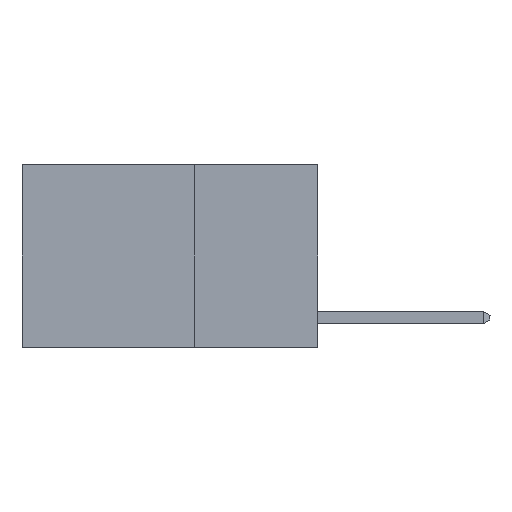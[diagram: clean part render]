
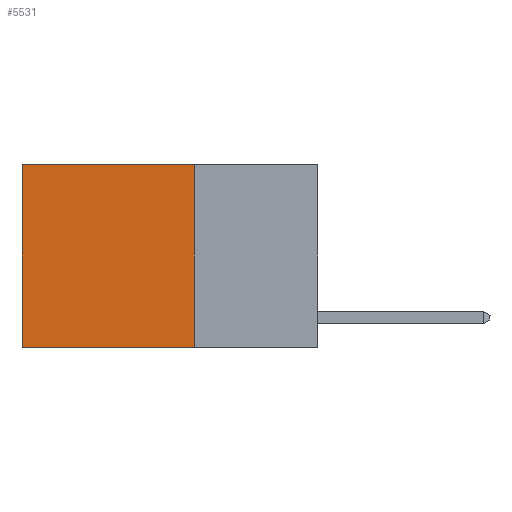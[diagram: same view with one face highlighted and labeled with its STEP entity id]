
A CAD part, left-side view. The second image highlights one B-rep face of the part: STEP entity #5531.
In plain terms, the highlighted planar face has unit normal (-1, 0, 0).
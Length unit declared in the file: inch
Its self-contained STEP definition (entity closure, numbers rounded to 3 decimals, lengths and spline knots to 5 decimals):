
#133 = LINE ( 'NONE', #4720, #2560 ) ;
#570 = EDGE_CURVE ( 'NONE', #7562, #9712, #12579, .T. ) ;
#711 = CARTESIAN_POINT ( 'NONE',  ( 0.2625, 0.6, 0. ) ) ;
#1269 = CARTESIAN_POINT ( 'NONE',  ( 0.2625, 0.6, -0.37 ) ) ;
#2114 = EDGE_CURVE ( 'NONE', #3166, #11554, #12125, .T. ) ;
#2398 = DIRECTION ( 'NONE',  ( 0., 0., -1. ) ) ;
#2560 = VECTOR ( 'NONE', #13889, 39.37008 ) ;
#3121 = DIRECTION ( 'NONE',  ( 0., 0., -1. ) ) ;
#3166 = VERTEX_POINT ( 'NONE', #5703 ) ;
#3882 = DIRECTION ( 'NONE',  ( 0., 1., 0. ) ) ;
#3989 = VECTOR ( 'NONE', #3121, 39.37008 ) ;
#4628 = PLANE ( 'NONE',  #12241 ) ;
#4720 = CARTESIAN_POINT ( 'NONE',  ( 0.2625, 0.25, -0.37 ) ) ;
#5531 = ADVANCED_FACE ( 'NONE', ( #12671 ), #4628, .F. ) ;
#5702 = EDGE_CURVE ( 'NONE', #7562, #3166, #8377, .T. ) ;
#5703 = CARTESIAN_POINT ( 'NONE',  ( 0.2625, 0.6, 0. ) ) ;
#5967 = CARTESIAN_POINT ( 'NONE',  ( 0.2625, 0.25, 0. ) ) ;
#6939 = CARTESIAN_POINT ( 'NONE',  ( 0.2625, 0.25, 0. ) ) ;
#7374 = EDGE_LOOP ( 'NONE', ( #14693, #11325, #11069, #13743 ) ) ;
#7562 = VERTEX_POINT ( 'NONE', #9446 ) ;
#7916 = DIRECTION ( 'NONE',  ( 0., 0., -1. ) ) ;
#8128 = VECTOR ( 'NONE', #3882, 39.37008 ) ;
#8377 = LINE ( 'NONE', #9724, #8128 ) ;
#8562 = VECTOR ( 'NONE', #7916, 39.37008 ) ;
#9446 = CARTESIAN_POINT ( 'NONE',  ( 0.2625, 0.25, 0. ) ) ;
#9712 = VERTEX_POINT ( 'NONE', #10630 ) ;
#9724 = CARTESIAN_POINT ( 'NONE',  ( 0.2625, 0.25, 0. ) ) ;
#10346 = DIRECTION ( 'NONE',  ( 1., 0., 0. ) ) ;
#10630 = CARTESIAN_POINT ( 'NONE',  ( 0.2625, 0.25, -0.37 ) ) ;
#11069 = ORIENTED_EDGE ( 'NONE', *, *, #570, .F. ) ;
#11325 = ORIENTED_EDGE ( 'NONE', *, *, #11556, .F. ) ;
#11554 = VERTEX_POINT ( 'NONE', #1269 ) ;
#11556 = EDGE_CURVE ( 'NONE', #9712, #11554, #133, .T. ) ;
#12125 = LINE ( 'NONE', #711, #3989 ) ;
#12241 = AXIS2_PLACEMENT_3D ( 'NONE', #5967, #10346, #2398 ) ;
#12579 = LINE ( 'NONE', #6939, #8562 ) ;
#12671 = FACE_OUTER_BOUND ( 'NONE', #7374, .T. ) ;
#13743 = ORIENTED_EDGE ( 'NONE', *, *, #5702, .T. ) ;
#13889 = DIRECTION ( 'NONE',  ( 0., 1., 0. ) ) ;
#14693 = ORIENTED_EDGE ( 'NONE', *, *, #2114, .T. ) ;
